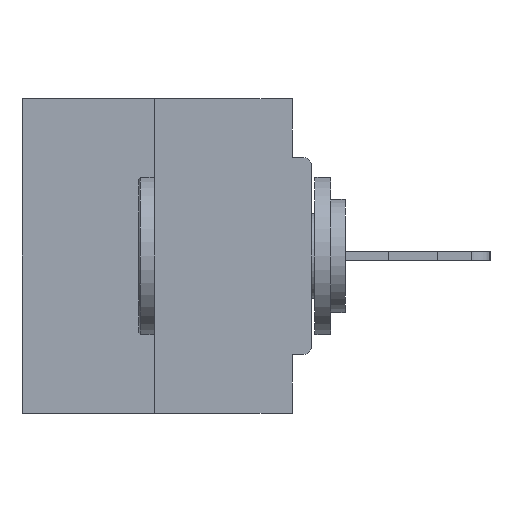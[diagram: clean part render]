
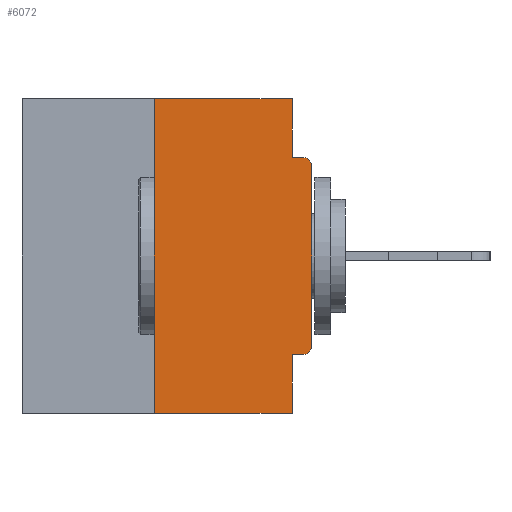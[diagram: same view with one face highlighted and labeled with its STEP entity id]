
A CAD part, left-side view. The second image highlights one B-rep face of the part: STEP entity #6072.
In plain terms, the highlighted planar face has unit normal (-1, 0, 0).
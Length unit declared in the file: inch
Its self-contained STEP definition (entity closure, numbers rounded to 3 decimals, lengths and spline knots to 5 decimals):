
#230 = CARTESIAN_POINT ( 'NONE',  ( 0., 0.25, 0. ) ) ;
#1660 = CIRCLE ( 'NONE', #23568, 0.015 ) ;
#2465 = VERTEX_POINT ( 'NONE', #21874 ) ;
#2469 = EDGE_CURVE ( 'NONE', #12791, #3580, #30706, .T. ) ;
#3096 = EDGE_CURVE ( 'NONE', #34295, #22143, #20816, .T. ) ;
#3580 = VERTEX_POINT ( 'NONE', #23508 ) ;
#4047 = DIRECTION ( 'NONE',  ( 0., 0., 1. ) ) ;
#4539 = CARTESIAN_POINT ( 'NONE',  ( 0., 0.031, 0. ) ) ;
#4604 = VERTEX_POINT ( 'NONE', #4539 ) ;
#4913 = CARTESIAN_POINT ( 'NONE',  ( 0., 0.46, 0. ) ) ;
#5093 = EDGE_LOOP ( 'NONE', ( #26437, #21053, #14853, #32917, #11583, #35661, #18352, #16259, #12512, #15750 ) ) ;
#5540 = CIRCLE ( 'NONE', #36838, 0.015 ) ;
#5610 = DIRECTION ( 'NONE',  ( 0., -1., 0. ) ) ;
#5853 = DIRECTION ( 'NONE',  ( 0., 0., -1. ) ) ;
#6072 = ADVANCED_FACE ( 'NONE', ( #25885 ), #37863, .F. ) ;
#6672 = EDGE_CURVE ( 'NONE', #3580, #2465, #1660, .T. ) ;
#8525 = VERTEX_POINT ( 'NONE', #31632 ) ;
#9424 = VECTOR ( 'NONE', #34916, 39.37008 ) ;
#9553 = EDGE_CURVE ( 'NONE', #34295, #11286, #32451, .T. ) ;
#10828 = LINE ( 'NONE', #22776, #37857 ) ;
#11188 = CARTESIAN_POINT ( 'NONE',  ( 0., 0.46, 0. ) ) ;
#11286 = VERTEX_POINT ( 'NONE', #20442 ) ;
#11581 = VECTOR ( 'NONE', #17479, 39.37008 ) ;
#11583 = ORIENTED_EDGE ( 'NONE', *, *, #29384, .F. ) ;
#11722 = CARTESIAN_POINT ( 'NONE',  ( 0., 0.031, 0. ) ) ;
#12512 = ORIENTED_EDGE ( 'NONE', *, *, #20695, .F. ) ;
#12791 = VERTEX_POINT ( 'NONE', #31031 ) ;
#13435 = DIRECTION ( 'NONE',  ( 0., 1., 0. ) ) ;
#14525 = VERTEX_POINT ( 'NONE', #38670 ) ;
#14853 = ORIENTED_EDGE ( 'NONE', *, *, #9553, .T. ) ;
#15750 = ORIENTED_EDGE ( 'NONE', *, *, #33779, .F. ) ;
#16031 = AXIS2_PLACEMENT_3D ( 'NONE', #4913, #17238, #38451 ) ;
#16259 = ORIENTED_EDGE ( 'NONE', *, *, #6672, .T. ) ;
#16367 = VERTEX_POINT ( 'NONE', #34458 ) ;
#16966 = VECTOR ( 'NONE', #23475, 39.37008 ) ;
#17238 = DIRECTION ( 'NONE',  ( 1., 0., 0. ) ) ;
#17479 = DIRECTION ( 'NONE',  ( 0., 0., 1. ) ) ;
#17975 = DIRECTION ( 'NONE',  ( -1., 0., 0. ) ) ;
#17983 = LINE ( 'NONE', #11722, #34942 ) ;
#18352 = ORIENTED_EDGE ( 'NONE', *, *, #2469, .T. ) ;
#20442 = CARTESIAN_POINT ( 'NONE',  ( 0., 0.031, -0.5 ) ) ;
#20695 = EDGE_CURVE ( 'NONE', #14525, #2465, #25656, .T. ) ;
#20816 = LINE ( 'NONE', #230, #11581 ) ;
#20878 = CARTESIAN_POINT ( 'NONE',  ( 0., 0.25, -0.5 ) ) ;
#20913 = DIRECTION ( 'NONE',  ( 0., 0., -1. ) ) ;
#21053 = ORIENTED_EDGE ( 'NONE', *, *, #3096, .F. ) ;
#21874 = CARTESIAN_POINT ( 'NONE',  ( 0., 0.015, -0.0935 ) ) ;
#22143 = VERTEX_POINT ( 'NONE', #38148 ) ;
#22253 = LINE ( 'NONE', #31086, #37944 ) ;
#22776 = CARTESIAN_POINT ( 'NONE',  ( 0., 0.031, -0.5 ) ) ;
#23078 = CARTESIAN_POINT ( 'NONE',  ( 0., 0.015, -0.3915 ) ) ;
#23475 = DIRECTION ( 'NONE',  ( 0., -1., 0. ) ) ;
#23508 = CARTESIAN_POINT ( 'NONE',  ( 0., 0., -0.1085 ) ) ;
#23568 = AXIS2_PLACEMENT_3D ( 'NONE', #35446, #17975, #20913 ) ;
#24905 = VECTOR ( 'NONE', #4047, 39.37008 ) ;
#25656 = LINE ( 'NONE', #29168, #16966 ) ;
#25885 = FACE_OUTER_BOUND ( 'NONE', #5093, .T. ) ;
#26437 = ORIENTED_EDGE ( 'NONE', *, *, #36374, .F. ) ;
#28152 = EDGE_CURVE ( 'NONE', #16367, #11286, #10828, .T. ) ;
#29168 = CARTESIAN_POINT ( 'NONE',  ( 0., 0., -0.0935 ) ) ;
#29384 = EDGE_CURVE ( 'NONE', #8525, #16367, #22253, .T. ) ;
#30706 = LINE ( 'NONE', #30904, #24905 ) ;
#30904 = CARTESIAN_POINT ( 'NONE',  ( 0., 0., 0. ) ) ;
#31031 = CARTESIAN_POINT ( 'NONE',  ( 0., 0., -0.3915 ) ) ;
#31086 = CARTESIAN_POINT ( 'NONE',  ( 0., 0., -0.4065 ) ) ;
#31341 = DIRECTION ( 'NONE',  ( -1., 0., 0. ) ) ;
#31606 = DIRECTION ( 'NONE',  ( 0., 0., -1. ) ) ;
#31632 = CARTESIAN_POINT ( 'NONE',  ( 0., 0.015, -0.4065 ) ) ;
#32114 = DIRECTION ( 'NONE',  ( 0., 0., -1. ) ) ;
#32451 = LINE ( 'NONE', #35408, #37474 ) ;
#32758 = LINE ( 'NONE', #11188, #9424 ) ;
#32917 = ORIENTED_EDGE ( 'NONE', *, *, #28152, .F. ) ;
#33736 = EDGE_CURVE ( 'NONE', #8525, #12791, #5540, .T. ) ;
#33779 = EDGE_CURVE ( 'NONE', #4604, #14525, #17983, .T. ) ;
#34295 = VERTEX_POINT ( 'NONE', #20878 ) ;
#34458 = CARTESIAN_POINT ( 'NONE',  ( 0., 0.031, -0.4065 ) ) ;
#34916 = DIRECTION ( 'NONE',  ( 0., -1., 0. ) ) ;
#34942 = VECTOR ( 'NONE', #5853, 39.37008 ) ;
#35408 = CARTESIAN_POINT ( 'NONE',  ( 0., 0.46, -0.5 ) ) ;
#35446 = CARTESIAN_POINT ( 'NONE',  ( 0., 0.015, -0.1085 ) ) ;
#35661 = ORIENTED_EDGE ( 'NONE', *, *, #33736, .T. ) ;
#36374 = EDGE_CURVE ( 'NONE', #22143, #4604, #32758, .T. ) ;
#36838 = AXIS2_PLACEMENT_3D ( 'NONE', #23078, #31341, #32114 ) ;
#37474 = VECTOR ( 'NONE', #5610, 39.37008 ) ;
#37857 = VECTOR ( 'NONE', #31606, 39.37008 ) ;
#37863 = PLANE ( 'NONE',  #16031 ) ;
#37944 = VECTOR ( 'NONE', #13435, 39.37008 ) ;
#38148 = CARTESIAN_POINT ( 'NONE',  ( 0., 0.25, 0. ) ) ;
#38451 = DIRECTION ( 'NONE',  ( 0., 0., -1. ) ) ;
#38670 = CARTESIAN_POINT ( 'NONE',  ( 0., 0.031, -0.0935 ) ) ;
